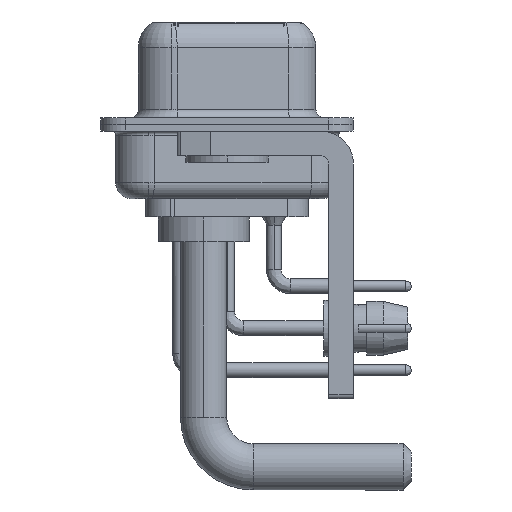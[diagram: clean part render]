
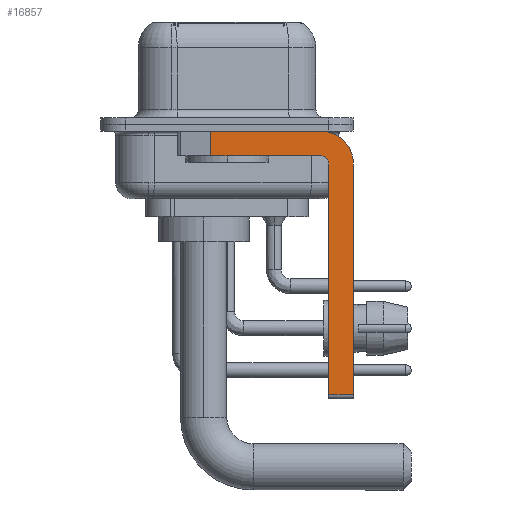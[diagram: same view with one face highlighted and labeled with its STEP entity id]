
A CAD part, left-side view. The second image highlights one B-rep face of the part: STEP entity #16857.
In plain terms, the highlighted planar face has unit normal (-1, 0, 0).
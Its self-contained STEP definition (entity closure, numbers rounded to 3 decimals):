
#57 = EDGE_CURVE ( 'NONE', #29374, #15815, #13537, .T. ) ;
#259 = CIRCLE ( 'NONE', #16665, 0.5 ) ;
#534 = ORIENTED_EDGE ( 'NONE', *, *, #57, .T. ) ;
#1036 = AXIS2_PLACEMENT_3D ( 'NONE', #14633, #16721, #14940 ) ;
#1559 = LINE ( 'NONE', #16324, #26599 ) ;
#1634 = AXIS2_PLACEMENT_3D ( 'NONE', #9683, #14635, #2437 ) ;
#1732 = DIRECTION ( 'NONE',  ( 0., -1., 0. ) ) ;
#2281 = FACE_OUTER_BOUND ( 'NONE', #23745, .T. ) ;
#2319 = ORIENTED_EDGE ( 'NONE', *, *, #12928, .F. ) ;
#2437 = DIRECTION ( 'NONE',  ( 0., 0., -1. ) ) ;
#2909 = DIRECTION ( 'NONE',  ( -1., 0., 0. ) ) ;
#4134 = CARTESIAN_POINT ( 'NONE',  ( -2.9, -6.15, -16.35 ) ) ;
#4163 = ORIENTED_EDGE ( 'NONE', *, *, #10666, .F. ) ;
#4280 = CARTESIAN_POINT ( 'NONE',  ( -2.9, -6.15, -2.4 ) ) ;
#4609 = VERTEX_POINT ( 'NONE', #26675 ) ;
#5551 = VERTEX_POINT ( 'NONE', #10239 ) ;
#6154 = DIRECTION ( 'NONE',  ( 0., -1., 0. ) ) ;
#6854 = DIRECTION ( 'NONE',  ( 0., 1., 0. ) ) ;
#8210 = VECTOR ( 'NONE', #15767, 1000. ) ;
#8531 = CARTESIAN_POINT ( 'NONE',  ( -2.9, -5.65, -2.4 ) ) ;
#8689 = VERTEX_POINT ( 'NONE', #4280 ) ;
#8773 = ORIENTED_EDGE ( 'NONE', *, *, #14008, .F. ) ;
#9683 = CARTESIAN_POINT ( 'NONE',  ( -2.9, -5.65, -2.4 ) ) ;
#9919 = ORIENTED_EDGE ( 'NONE', *, *, #22573, .T. ) ;
#10239 = CARTESIAN_POINT ( 'NONE',  ( -2.9, -7.65, -2.4 ) ) ;
#10583 = CARTESIAN_POINT ( 'NONE',  ( -2.9, -6.15, -16.6 ) ) ;
#10666 = EDGE_CURVE ( 'NONE', #5551, #15689, #21218, .T. ) ;
#11563 = ORIENTED_EDGE ( 'NONE', *, *, #20082, .F. ) ;
#12024 = VECTOR ( 'NONE', #17328, 1000. ) ;
#12928 = EDGE_CURVE ( 'NONE', #29332, #15815, #1559, .T. ) ;
#13537 = LINE ( 'NONE', #30708, #13552 ) ;
#13552 = VECTOR ( 'NONE', #27666, 1000. ) ;
#14008 = EDGE_CURVE ( 'NONE', #4609, #5551, #26138, .T. ) ;
#14348 = ORIENTED_EDGE ( 'NONE', *, *, #18959, .F. ) ;
#14633 = CARTESIAN_POINT ( 'NONE',  ( -2.9, -5.65, -2.4 ) ) ;
#14635 = DIRECTION ( 'NONE',  ( 1., 0., 0. ) ) ;
#14940 = DIRECTION ( 'NONE',  ( 0., 0., -1. ) ) ;
#15281 = VECTOR ( 'NONE', #6154, 1000. ) ;
#15689 = VERTEX_POINT ( 'NONE', #16421 ) ;
#15767 = DIRECTION ( 'NONE',  ( 0., 0., -1. ) ) ;
#15815 = VERTEX_POINT ( 'NONE', #18625 ) ;
#16240 = VERTEX_POINT ( 'NONE', #4134 ) ;
#16324 = CARTESIAN_POINT ( 'NONE',  ( -2.9, -5.65, -1.9 ) ) ;
#16421 = CARTESIAN_POINT ( 'NONE',  ( -2.9, -7.65, -16.35 ) ) ;
#16508 = CARTESIAN_POINT ( 'NONE',  ( -2.9, 0.978, -0.4 ) ) ;
#16665 = AXIS2_PLACEMENT_3D ( 'NONE', #8531, #2909, #27291 ) ;
#16721 = DIRECTION ( 'NONE',  ( 1., 0., 0. ) ) ;
#16857 = ADVANCED_FACE ( 'NONE', ( #2281 ), #21852, .F. ) ;
#17328 = DIRECTION ( 'NONE',  ( 0., 0., 1. ) ) ;
#18348 = CARTESIAN_POINT ( 'NONE',  ( -2.9, -7.65, -2.4 ) ) ;
#18363 = LINE ( 'NONE', #22849, #15281 ) ;
#18625 = CARTESIAN_POINT ( 'NONE',  ( -2.9, 0.978, -1.9 ) ) ;
#18959 = EDGE_CURVE ( 'NONE', #29374, #4609, #23708, .T. ) ;
#19986 = EDGE_CURVE ( 'NONE', #8689, #29332, #259, .T. ) ;
#20082 = EDGE_CURVE ( 'NONE', #16240, #8689, #20516, .T. ) ;
#20221 = VECTOR ( 'NONE', #1732, 1000. ) ;
#20516 = LINE ( 'NONE', #10583, #12024 ) ;
#21218 = LINE ( 'NONE', #18348, #8210 ) ;
#21852 = PLANE ( 'NONE',  #1634 ) ;
#22573 = EDGE_CURVE ( 'NONE', #16240, #15689, #18363, .T. ) ;
#22849 = CARTESIAN_POINT ( 'NONE',  ( -2.9, -5.65, -16.35 ) ) ;
#23708 = LINE ( 'NONE', #23873, #20221 ) ;
#23745 = EDGE_LOOP ( 'NONE', ( #14348, #534, #2319, #29836, #11563, #9919, #4163, #8773 ) ) ;
#23873 = CARTESIAN_POINT ( 'NONE',  ( -2.9, 3., -0.4 ) ) ;
#23885 = CARTESIAN_POINT ( 'NONE',  ( -2.9, -5.65, -1.9 ) ) ;
#26138 = CIRCLE ( 'NONE', #1036, 2. ) ;
#26599 = VECTOR ( 'NONE', #6854, 1000. ) ;
#26675 = CARTESIAN_POINT ( 'NONE',  ( -2.9, -5.65, -0.4 ) ) ;
#27291 = DIRECTION ( 'NONE',  ( 0., 0., 1. ) ) ;
#27666 = DIRECTION ( 'NONE',  ( 0., 0., -1. ) ) ;
#29332 = VERTEX_POINT ( 'NONE', #23885 ) ;
#29374 = VERTEX_POINT ( 'NONE', #16508 ) ;
#29836 = ORIENTED_EDGE ( 'NONE', *, *, #19986, .F. ) ;
#30708 = CARTESIAN_POINT ( 'NONE',  ( -2.9, 0.978, -1.9 ) ) ;
